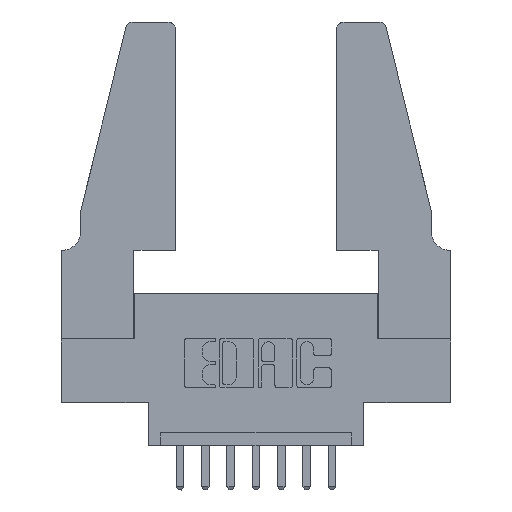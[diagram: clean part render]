
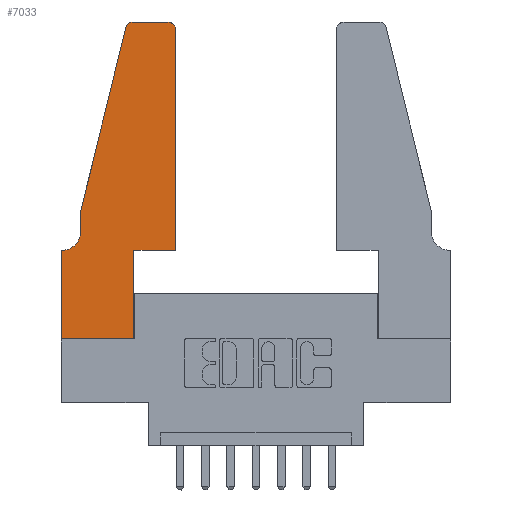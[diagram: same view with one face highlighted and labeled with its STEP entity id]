
A CAD part, top view. The second image highlights one B-rep face of the part: STEP entity #7033.
In plain terms, the highlighted planar face has unit normal (0, 0, 1).
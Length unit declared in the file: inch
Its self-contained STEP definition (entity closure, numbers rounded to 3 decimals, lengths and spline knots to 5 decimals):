
#128 = AXIS2_PLACEMENT_3D ( 'NONE', #5648, #4787, #1992 ) ;
#137 = CARTESIAN_POINT ( 'NONE',  ( 0., 0., 0.37 ) ) ;
#143 = VECTOR ( 'NONE', #6533, 39.37008 ) ;
#207 = CARTESIAN_POINT ( 'NONE',  ( 0.0755, 0.5, 0.37 ) ) ;
#211 = EDGE_CURVE ( 'NONE', #2429, #2191, #7975, .T. ) ;
#233 = CARTESIAN_POINT ( 'NONE',  ( 0.4505, 1.22, 0.37 ) ) ;
#237 = CARTESIAN_POINT ( 'NONE',  ( 0., 0.35, 0.37 ) ) ;
#260 = DIRECTION ( 'NONE',  ( -1., 0., 0. ) ) ;
#461 = LINE ( 'NONE', #207, #10461 ) ;
#577 = ORIENTED_EDGE ( 'NONE', *, *, #8549, .T. ) ;
#694 = EDGE_CURVE ( 'NONE', #3165, #12154, #461, .T. ) ;
#892 = CARTESIAN_POINT ( 'NONE',  ( 0., 0., 0.37 ) ) ;
#988 = VECTOR ( 'NONE', #4432, 39.37008 ) ;
#1173 = EDGE_CURVE ( 'NONE', #3379, #8553, #4478, .T. ) ;
#1430 = CARTESIAN_POINT ( 'NONE',  ( 0.4505, 0.35, 0.37 ) ) ;
#1508 = LINE ( 'NONE', #4959, #8967 ) ;
#1532 = DIRECTION ( 'NONE',  ( 1., 0., 0. ) ) ;
#1684 = VERTEX_POINT ( 'NONE', #7510 ) ;
#1700 = CIRCLE ( 'NONE', #4815, 0.07 ) ;
#1737 = VERTEX_POINT ( 'NONE', #233 ) ;
#1992 = DIRECTION ( 'NONE',  ( 1., 0., 0. ) ) ;
#2026 = EDGE_CURVE ( 'NONE', #1737, #6038, #7130, .T. ) ;
#2191 = VERTEX_POINT ( 'NONE', #4364 ) ;
#2222 = LINE ( 'NONE', #892, #5215 ) ;
#2272 = LINE ( 'NONE', #6650, #6457 ) ;
#2406 = CARTESIAN_POINT ( 'NONE',  ( 0.2865, 0.35, 0.37 ) ) ;
#2429 = VERTEX_POINT ( 'NONE', #10440 ) ;
#2448 = CARTESIAN_POINT ( 'NONE',  ( 0.0055, 0.42, 0.37 ) ) ;
#2879 = DIRECTION ( 'NONE',  ( 0., -1., 0. ) ) ;
#3025 = EDGE_CURVE ( 'NONE', #10369, #10829, #3400, .T. ) ;
#3164 = ORIENTED_EDGE ( 'NONE', *, *, #10446, .T. ) ;
#3165 = VERTEX_POINT ( 'NONE', #10171 ) ;
#3379 = VERTEX_POINT ( 'NONE', #4615 ) ;
#3400 = CIRCLE ( 'NONE', #5992, 0.03 ) ;
#3438 = CARTESIAN_POINT ( 'NONE',  ( 0.4205, 1.22, 0.37 ) ) ;
#3492 = ORIENTED_EDGE ( 'NONE', *, *, #694, .T. ) ;
#3923 = CARTESIAN_POINT ( 'NONE',  ( 0.0755, 0.42, 0.37 ) ) ;
#3983 = ORIENTED_EDGE ( 'NONE', *, *, #7156, .T. ) ;
#4364 = CARTESIAN_POINT ( 'NONE',  ( 0.4505, 0.35, 0.37 ) ) ;
#4432 = DIRECTION ( 'NONE',  ( 1., 0., 0. ) ) ;
#4478 = LINE ( 'NONE', #10409, #8797 ) ;
#4523 = CARTESIAN_POINT ( 'NONE',  ( 0.4205, 1.25, 0.37 ) ) ;
#4615 = CARTESIAN_POINT ( 'NONE',  ( 0.0055, 0.35, 0.37 ) ) ;
#4787 = DIRECTION ( 'NONE',  ( 0., 0., 1. ) ) ;
#4815 = AXIS2_PLACEMENT_3D ( 'NONE', #2448, #6240, #6326 ) ;
#4925 = EDGE_CURVE ( 'NONE', #12154, #3379, #1700, .T. ) ;
#4959 = CARTESIAN_POINT ( 'NONE',  ( 0.2605, 1.25, 0.37 ) ) ;
#5100 = ORIENTED_EDGE ( 'NONE', *, *, #1173, .T. ) ;
#5215 = VECTOR ( 'NONE', #10474, 39.37008 ) ;
#5227 = ORIENTED_EDGE ( 'NONE', *, *, #10926, .T. ) ;
#5355 = DIRECTION ( 'NONE',  ( 1., 0., 0. ) ) ;
#5648 = CARTESIAN_POINT ( 'NONE',  ( 0., 0.35, 0.37 ) ) ;
#5658 = AXIS2_PLACEMENT_3D ( 'NONE', #3438, #12118, #5355 ) ;
#5903 = ORIENTED_EDGE ( 'NONE', *, *, #211, .T. ) ;
#5932 = CARTESIAN_POINT ( 'NONE',  ( 0.25487, 1.22718, 0.37 ) ) ;
#5992 = AXIS2_PLACEMENT_3D ( 'NONE', #7224, #9334, #1532 ) ;
#6038 = VERTEX_POINT ( 'NONE', #4523 ) ;
#6240 = DIRECTION ( 'NONE',  ( 0., 0., -1. ) ) ;
#6326 = DIRECTION ( 'NONE',  ( -1., 0., 0. ) ) ;
#6455 = EDGE_CURVE ( 'NONE', #2191, #1737, #7329, .T. ) ;
#6457 = VECTOR ( 'NONE', #2879, 39.37008 ) ;
#6533 = DIRECTION ( 'NONE',  ( -0.239, -0.971, 0. ) ) ;
#6613 = DIRECTION ( 'NONE',  ( 0., 1., 0. ) ) ;
#6650 = CARTESIAN_POINT ( 'NONE',  ( 0., 0., 0.37 ) ) ;
#6840 = ORIENTED_EDGE ( 'NONE', *, *, #4925, .T. ) ;
#7033 = ADVANCED_FACE ( 'NONE', ( #9786 ), #8588, .T. ) ;
#7130 = CIRCLE ( 'NONE', #5658, 0.03 ) ;
#7156 = EDGE_CURVE ( 'NONE', #1684, #2429, #11749, .T. ) ;
#7224 = CARTESIAN_POINT ( 'NONE',  ( 0.284, 1.22, 0.37 ) ) ;
#7329 = LINE ( 'NONE', #1430, #10024 ) ;
#7510 = CARTESIAN_POINT ( 'NONE',  ( 0.2865, 0., 0.37 ) ) ;
#7975 = LINE ( 'NONE', #10153, #988 ) ;
#8064 = DIRECTION ( 'NONE',  ( 0., 1., 0. ) ) ;
#8297 = VERTEX_POINT ( 'NONE', #137 ) ;
#8549 = EDGE_CURVE ( 'NONE', #8553, #8297, #2272, .T. ) ;
#8553 = VERTEX_POINT ( 'NONE', #237 ) ;
#8588 = PLANE ( 'NONE',  #128 ) ;
#8790 = DIRECTION ( 'NONE',  ( 0., -1., 0. ) ) ;
#8797 = VECTOR ( 'NONE', #12200, 39.37008 ) ;
#8967 = VECTOR ( 'NONE', #260, 39.37008 ) ;
#9334 = DIRECTION ( 'NONE',  ( 0., 0., 1. ) ) ;
#9786 = FACE_OUTER_BOUND ( 'NONE', #11774, .T. ) ;
#10024 = VECTOR ( 'NONE', #6613, 39.37008 ) ;
#10153 = CARTESIAN_POINT ( 'NONE',  ( 0.4505, 0.35, 0.37 ) ) ;
#10171 = CARTESIAN_POINT ( 'NONE',  ( 0.0755, 0.5, 0.37 ) ) ;
#10215 = ORIENTED_EDGE ( 'NONE', *, *, #6455, .T. ) ;
#10369 = VERTEX_POINT ( 'NONE', #12097 ) ;
#10409 = CARTESIAN_POINT ( 'NONE',  ( 0.0755, 0.35, 0.37 ) ) ;
#10440 = CARTESIAN_POINT ( 'NONE',  ( 0.2865, 0.35, 0.37 ) ) ;
#10446 = EDGE_CURVE ( 'NONE', #6038, #10369, #1508, .T. ) ;
#10461 = VECTOR ( 'NONE', #8790, 39.37008 ) ;
#10474 = DIRECTION ( 'NONE',  ( 1., 0., 0. ) ) ;
#10501 = ORIENTED_EDGE ( 'NONE', *, *, #10976, .T. ) ;
#10829 = VERTEX_POINT ( 'NONE', #5932 ) ;
#10921 = LINE ( 'NONE', #11334, #143 ) ;
#10926 = EDGE_CURVE ( 'NONE', #8297, #1684, #2222, .T. ) ;
#10976 = EDGE_CURVE ( 'NONE', #10829, #3165, #10921, .T. ) ;
#11009 = VECTOR ( 'NONE', #8064, 39.37008 ) ;
#11032 = ORIENTED_EDGE ( 'NONE', *, *, #2026, .T. ) ;
#11334 = CARTESIAN_POINT ( 'NONE',  ( 0.0755, 0.5, 0.37 ) ) ;
#11548 = ORIENTED_EDGE ( 'NONE', *, *, #3025, .T. ) ;
#11749 = LINE ( 'NONE', #2406, #11009 ) ;
#11774 = EDGE_LOOP ( 'NONE', ( #3164, #11548, #10501, #3492, #6840, #5100, #577, #5227, #3983, #5903, #10215, #11032 ) ) ;
#12097 = CARTESIAN_POINT ( 'NONE',  ( 0.284, 1.25, 0.37 ) ) ;
#12118 = DIRECTION ( 'NONE',  ( 0., 0., 1. ) ) ;
#12154 = VERTEX_POINT ( 'NONE', #3923 ) ;
#12200 = DIRECTION ( 'NONE',  ( -1., 0., 0. ) ) ;
